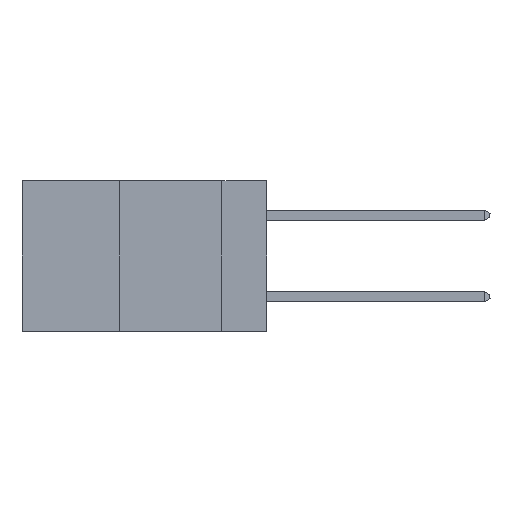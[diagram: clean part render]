
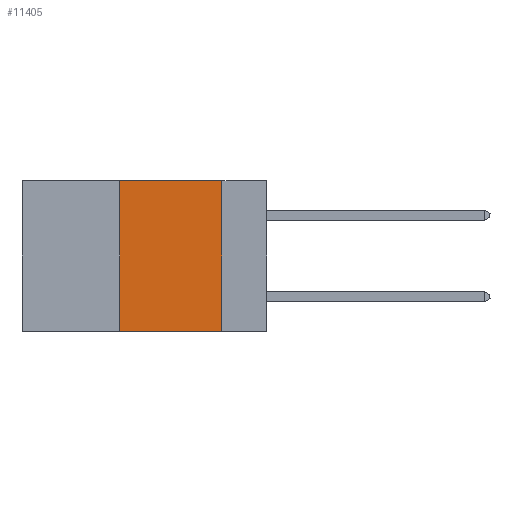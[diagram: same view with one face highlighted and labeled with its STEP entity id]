
A CAD part, left-side view. The second image highlights one B-rep face of the part: STEP entity #11405.
In plain terms, the highlighted planar face has unit normal (-1, 0, 0).
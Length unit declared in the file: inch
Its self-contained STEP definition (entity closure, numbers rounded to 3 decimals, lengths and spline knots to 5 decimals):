
#332 = EDGE_CURVE ( 'NONE', #8735, #7423, #9112, .T. ) ;
#486 = FACE_OUTER_BOUND ( 'NONE', #11265, .T. ) ;
#790 = EDGE_CURVE ( 'NONE', #8029, #9078, #2385, .T. ) ;
#1389 = CARTESIAN_POINT ( 'NONE',  ( 0., 0.11, 0. ) ) ;
#1433 = ORIENTED_EDGE ( 'NONE', *, *, #1492, .F. ) ;
#1492 = EDGE_CURVE ( 'NONE', #9078, #7423, #6446, .T. ) ;
#1550 = ORIENTED_EDGE ( 'NONE', *, *, #790, .F. ) ;
#2079 = CARTESIAN_POINT ( 'NONE',  ( 0., 0.6, 0. ) ) ;
#2385 = LINE ( 'NONE', #5279, #11669 ) ;
#2748 = CARTESIAN_POINT ( 'NONE',  ( 0., 0.36, 0. ) ) ;
#2984 = DIRECTION ( 'NONE',  ( 1., 0., 0. ) ) ;
#3470 = CARTESIAN_POINT ( 'NONE',  ( 0., 0.11, 0. ) ) ;
#3599 = EDGE_CURVE ( 'NONE', #8735, #8029, #4492, .T. ) ;
#4080 = DIRECTION ( 'NONE',  ( 0., 0., -1. ) ) ;
#4217 = ORIENTED_EDGE ( 'NONE', *, *, #3599, .F. ) ;
#4492 = LINE ( 'NONE', #2748, #9958 ) ;
#5279 = CARTESIAN_POINT ( 'NONE',  ( 0., 0.6, 0. ) ) ;
#6062 = VECTOR ( 'NONE', #7305, 39.37008 ) ;
#6446 = LINE ( 'NONE', #1389, #7708 ) ;
#6488 = CARTESIAN_POINT ( 'NONE',  ( 0., 0.11, -0.37 ) ) ;
#7073 = DIRECTION ( 'NONE',  ( 0., -1., 0. ) ) ;
#7305 = DIRECTION ( 'NONE',  ( 0., -1., 0. ) ) ;
#7423 = VERTEX_POINT ( 'NONE', #6488 ) ;
#7708 = VECTOR ( 'NONE', #4080, 39.37008 ) ;
#8029 = VERTEX_POINT ( 'NONE', #10288 ) ;
#8309 = AXIS2_PLACEMENT_3D ( 'NONE', #2079, #2984, #9224 ) ;
#8735 = VERTEX_POINT ( 'NONE', #10894 ) ;
#8952 = CARTESIAN_POINT ( 'NONE',  ( 0., 0.6, -0.37 ) ) ;
#9078 = VERTEX_POINT ( 'NONE', #3470 ) ;
#9112 = LINE ( 'NONE', #8952, #6062 ) ;
#9224 = DIRECTION ( 'NONE',  ( 0., 0., -1. ) ) ;
#9528 = ORIENTED_EDGE ( 'NONE', *, *, #332, .T. ) ;
#9958 = VECTOR ( 'NONE', #10037, 39.37008 ) ;
#10037 = DIRECTION ( 'NONE',  ( 0., 0., 1. ) ) ;
#10288 = CARTESIAN_POINT ( 'NONE',  ( 0., 0.36, 0. ) ) ;
#10894 = CARTESIAN_POINT ( 'NONE',  ( 0., 0.36, -0.37 ) ) ;
#11112 = PLANE ( 'NONE',  #8309 ) ;
#11265 = EDGE_LOOP ( 'NONE', ( #1433, #1550, #4217, #9528 ) ) ;
#11405 = ADVANCED_FACE ( 'NONE', ( #486 ), #11112, .F. ) ;
#11669 = VECTOR ( 'NONE', #7073, 39.37008 ) ;
